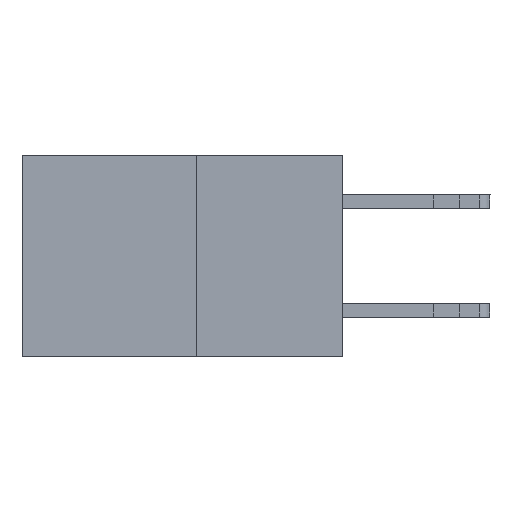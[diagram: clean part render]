
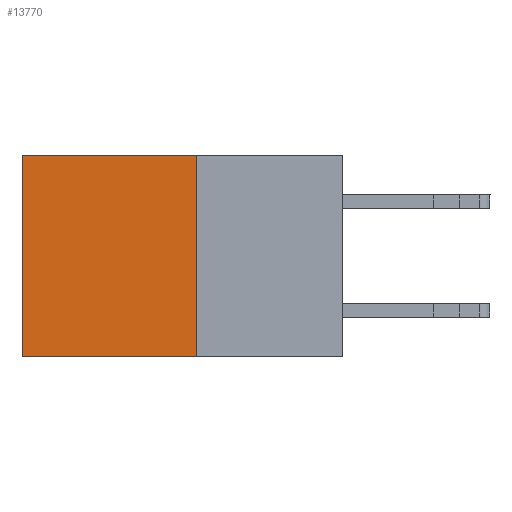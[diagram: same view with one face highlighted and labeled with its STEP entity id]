
A CAD part, left-side view. The second image highlights one B-rep face of the part: STEP entity #13770.
In plain terms, the highlighted planar face has unit normal (-1, 0, 0).
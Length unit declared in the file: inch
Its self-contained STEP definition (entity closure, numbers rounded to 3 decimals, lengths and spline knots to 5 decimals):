
#154 = ORIENTED_EDGE ( 'NONE', *, *, #1897, .T. ) ;
#588 = CARTESIAN_POINT ( 'NONE',  ( 0.277, 0.27, -0.37 ) ) ;
#1897 = EDGE_CURVE ( 'NONE', #16671, #2880, #9557, .T. ) ;
#2837 = EDGE_CURVE ( 'NONE', #2880, #12272, #10596, .T. ) ;
#2880 = VERTEX_POINT ( 'NONE', #8284 ) ;
#3192 = ORIENTED_EDGE ( 'NONE', *, *, #12954, .F. ) ;
#4966 = DIRECTION ( 'NONE',  ( 0., 0., -1. ) ) ;
#5468 = DIRECTION ( 'NONE',  ( 0., 1., 0. ) ) ;
#5621 = CARTESIAN_POINT ( 'NONE',  ( 0.277, 0.27, -0.37 ) ) ;
#6117 = PLANE ( 'NONE',  #9373 ) ;
#6593 = VERTEX_POINT ( 'NONE', #5621 ) ;
#6774 = DIRECTION ( 'NONE',  ( 0., 0., -1. ) ) ;
#7502 = DIRECTION ( 'NONE',  ( 0., 0., -1. ) ) ;
#8284 = CARTESIAN_POINT ( 'NONE',  ( 0.277, 0.59, 0. ) ) ;
#8409 = VECTOR ( 'NONE', #4966, 39.37008 ) ;
#9373 = AXIS2_PLACEMENT_3D ( 'NONE', #588, #10478, #7502 ) ;
#9378 = VECTOR ( 'NONE', #5468, 39.37008 ) ;
#9557 = LINE ( 'NONE', #18124, #9378 ) ;
#9642 = VECTOR ( 'NONE', #11387, 39.37008 ) ;
#10478 = DIRECTION ( 'NONE',  ( 1., 0., 0. ) ) ;
#10596 = LINE ( 'NONE', #17618, #8409 ) ;
#10876 = EDGE_LOOP ( 'NONE', ( #13140, #3192, #15987, #154 ) ) ;
#11387 = DIRECTION ( 'NONE',  ( 0., 1., 0. ) ) ;
#11417 = VECTOR ( 'NONE', #6774, 39.37008 ) ;
#12272 = VERTEX_POINT ( 'NONE', #17797 ) ;
#12633 = CARTESIAN_POINT ( 'NONE',  ( 0.277, 0.27, 0. ) ) ;
#12954 = EDGE_CURVE ( 'NONE', #6593, #12272, #14592, .T. ) ;
#13140 = ORIENTED_EDGE ( 'NONE', *, *, #2837, .T. ) ;
#13204 = EDGE_CURVE ( 'NONE', #16671, #6593, #15181, .T. ) ;
#13770 = ADVANCED_FACE ( 'NONE', ( #15731 ), #6117, .F. ) ;
#13812 = CARTESIAN_POINT ( 'NONE',  ( 0.277, 0.27, -0.37 ) ) ;
#14592 = LINE ( 'NONE', #15895, #9642 ) ;
#15181 = LINE ( 'NONE', #13812, #11417 ) ;
#15731 = FACE_OUTER_BOUND ( 'NONE', #10876, .T. ) ;
#15895 = CARTESIAN_POINT ( 'NONE',  ( 0.277, 0.27, -0.37 ) ) ;
#15987 = ORIENTED_EDGE ( 'NONE', *, *, #13204, .F. ) ;
#16671 = VERTEX_POINT ( 'NONE', #12633 ) ;
#17618 = CARTESIAN_POINT ( 'NONE',  ( 0.277, 0.59, -0.37 ) ) ;
#17797 = CARTESIAN_POINT ( 'NONE',  ( 0.277, 0.59, -0.37 ) ) ;
#18124 = CARTESIAN_POINT ( 'NONE',  ( 0.277, 0.27, 0. ) ) ;
